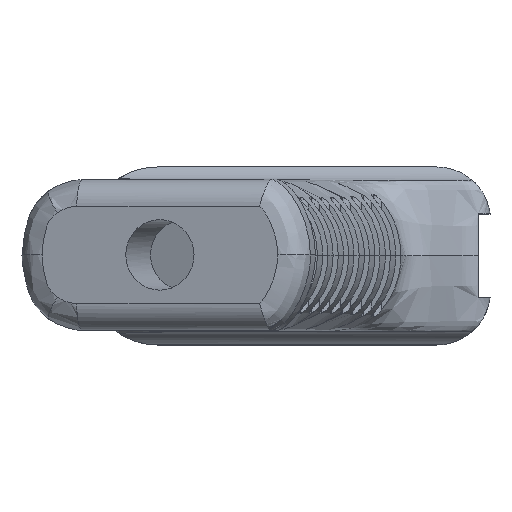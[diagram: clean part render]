
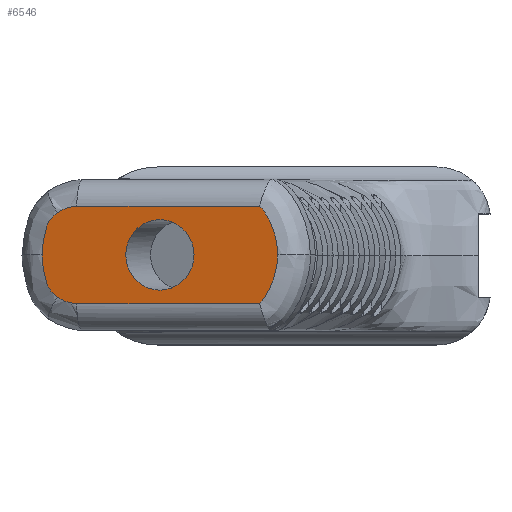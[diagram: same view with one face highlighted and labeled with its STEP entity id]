
A CAD part, top view. The second image highlights one B-rep face of the part: STEP entity #6546.
In plain terms, the highlighted planar face has unit normal (-0.249, 0, 0.969).
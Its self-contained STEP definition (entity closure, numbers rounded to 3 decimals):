
#104=B_SPLINE_CURVE_WITH_KNOTS('',3,(#9156,#9157,#9158,#9159,#9160,#9161,
#9162,#9163,#9164,#9165,#9166,#9167,#9168,#9169,#9170,#9171,#9172,#9173,
#9174,#9175,#9176,#9177,#9178),.UNSPECIFIED.,.F.,.F.,(4,1,1,1,1,1,2,1,1,
1,1,1,2,1,2,1,1,4),(0.,0.054,0.161,
0.214,0.268,0.321,0.375,
0.444,0.513,0.582,0.651,
0.685,0.72,0.745,0.761,
0.775,0.788,0.793),.UNSPECIFIED.);
#105=B_SPLINE_CURVE_WITH_KNOTS('',3,(#9180,#9181,#9182,#9183,#9184,#9185,
#9186,#9187,#9188,#9189,#9190,#9191,#9192,#9193,#9194),.UNSPECIFIED.,.F.,
 .F.,(4,1,1,1,1,1,1,1,2,1,1,4),(0.035,0.044,0.066,
0.08,0.108,0.223,0.338,
0.395,0.453,0.578,0.703,
0.828),.UNSPECIFIED.);
#106=B_SPLINE_CURVE_WITH_KNOTS('',3,(#9198,#9199,#9200,#9201,#9202,#9203),
 .UNSPECIFIED.,.F.,.F.,(4,2,4),(-0.321,-0.296,-0.005),
 .UNSPECIFIED.);
#107=B_SPLINE_CURVE_WITH_KNOTS('',3,(#9205,#9206,#9207,#9208,#9209,#9210,
#9211,#9212),.UNSPECIFIED.,.F.,.F.,(4,1,2,1,4),(0.,0.25,0.438,
0.549,0.696),.UNSPECIFIED.);
#108=B_SPLINE_CURVE_WITH_KNOTS('',3,(#9214,#9215,#9216,#9217,#9218,#9219,
#9220),.UNSPECIFIED.,.F.,.F.,(4,1,2,4),(0.,0.148,0.26,
0.698),.UNSPECIFIED.);
#109=B_SPLINE_CURVE_WITH_KNOTS('',3,(#9221,#9222,#9223,#9224,#9225,#9226),
 .UNSPECIFIED.,.F.,.F.,(4,2,4),(-0.316,-0.025,
0.),.UNSPECIFIED.);
#658=FACE_BOUND('',#1186,.T.);
#667=CIRCLE('',#6907,5.25);
#814=FACE_OUTER_BOUND('',#1185,.T.);
#1185=EDGE_LOOP('',(#4716,#4717,#4718,#4719,#4720,#4721,#4722,#4723));
#1186=EDGE_LOOP('',(#4724));
#1679=LINE('',#9154,#2199);
#1680=LINE('',#9196,#2200);
#2199=VECTOR('',#7694,10.);
#2200=VECTOR('',#7695,10.);
#2630=VERTEX_POINT('',#8848);
#2690=VERTEX_POINT('',#9152);
#2691=VERTEX_POINT('',#9153);
#2692=VERTEX_POINT('',#9155);
#2693=VERTEX_POINT('',#9179);
#2694=VERTEX_POINT('',#9195);
#2695=VERTEX_POINT('',#9197);
#2696=VERTEX_POINT('',#9204);
#2697=VERTEX_POINT('',#9213);
#3358=EDGE_CURVE('',#2630,#2630,#667,.T.);
#3448=EDGE_CURVE('',#2690,#2691,#1679,.T.);
#3449=EDGE_CURVE('',#2692,#2690,#104,.T.);
#3450=EDGE_CURVE('',#2693,#2692,#105,.T.);
#3451=EDGE_CURVE('',#2694,#2693,#1680,.T.);
#3452=EDGE_CURVE('',#2695,#2694,#106,.T.);
#3453=EDGE_CURVE('',#2696,#2695,#107,.T.);
#3454=EDGE_CURVE('',#2697,#2696,#108,.T.);
#3455=EDGE_CURVE('',#2691,#2697,#109,.T.);
#4716=ORIENTED_EDGE('',*,*,#3448,.F.);
#4717=ORIENTED_EDGE('',*,*,#3449,.F.);
#4718=ORIENTED_EDGE('',*,*,#3450,.F.);
#4719=ORIENTED_EDGE('',*,*,#3451,.F.);
#4720=ORIENTED_EDGE('',*,*,#3452,.F.);
#4721=ORIENTED_EDGE('',*,*,#3453,.F.);
#4722=ORIENTED_EDGE('',*,*,#3454,.F.);
#4723=ORIENTED_EDGE('',*,*,#3455,.F.);
#4724=ORIENTED_EDGE('',*,*,#3358,.T.);
#6342=PLANE('',#6974);
#6546=ADVANCED_FACE('',(#814,#658),#6342,.F.);
#6907=AXIS2_PLACEMENT_3D('',#8849,#7508,#7509);
#6974=AXIS2_PLACEMENT_3D('',#9151,#7692,#7693);
#7508=DIRECTION('center_axis',(0.249,0.,-0.969));
#7509=DIRECTION('ref_axis',(0.,-1.,0.));
#7692=DIRECTION('center_axis',(0.249,0.,-0.969));
#7693=DIRECTION('ref_axis',(0.969,0.,0.249));
#7694=DIRECTION('',(-0.969,0.,-0.249));
#7695=DIRECTION('',(0.969,0.,0.249));
#8848=CARTESIAN_POINT('',(-49.151,-78.684,-18.57));
#8849=CARTESIAN_POINT('Origin',(-49.151,-83.934,-18.57));
#9151=CARTESIAN_POINT('Origin',(-81.64,-72.686,-26.907));
#9152=CARTESIAN_POINT('',(-34.333,-91.182,-14.767));
#9153=CARTESIAN_POINT('',(-61.522,-91.18,-21.745));
#9154=CARTESIAN_POINT('',(-52.784,-91.182,-19.502));
#9155=CARTESIAN_POINT('',(-31.61,-83.935,-14.069));
#9156=CARTESIAN_POINT('Ctrl Pts',(-31.61,-83.935,-14.069));
#9157=CARTESIAN_POINT('Ctrl Pts',(-31.61,-84.112,-14.069));
#9158=CARTESIAN_POINT('Ctrl Pts',(-31.625,-84.648,-14.072));
#9159=CARTESIAN_POINT('Ctrl Pts',(-31.699,-85.362,-14.091));
#9160=CARTESIAN_POINT('Ctrl Pts',(-31.825,-86.069,-14.124));
#9161=CARTESIAN_POINT('Ctrl Pts',(-31.945,-86.593,-14.154));
#9162=CARTESIAN_POINT('Ctrl Pts',(-32.089,-87.109,-14.192));
#9163=CARTESIAN_POINT('Ctrl Pts',(-32.201,-87.447,-14.22));
#9164=CARTESIAN_POINT('Ctrl Pts',(-32.34,-87.83,-14.256));
#9165=CARTESIAN_POINT('Ctrl Pts',(-32.504,-88.26,-14.298));
#9166=CARTESIAN_POINT('Ctrl Pts',(-32.777,-88.892,-14.368));
#9167=CARTESIAN_POINT('Ctrl Pts',(-33.083,-89.509,-14.447));
#9168=CARTESIAN_POINT('Ctrl Pts',(-33.368,-90.002,-14.52));
#9169=CARTESIAN_POINT('Ctrl Pts',(-33.623,-90.384,-14.585));
#9170=CARTESIAN_POINT('Ctrl Pts',(-33.761,-90.569,-14.62));
#9171=CARTESIAN_POINT('Ctrl Pts',(-33.884,-90.723,-14.652));
#9172=CARTESIAN_POINT('Ctrl Pts',(-33.972,-90.828,-14.675));
#9173=CARTESIAN_POINT('Ctrl Pts',(-34.065,-90.929,-14.699));
#9174=CARTESIAN_POINT('Ctrl Pts',(-34.133,-90.999,-14.716));
#9175=CARTESIAN_POINT('Ctrl Pts',(-34.195,-91.061,-14.732));
#9176=CARTESIAN_POINT('Ctrl Pts',(-34.273,-91.131,-14.752));
#9177=CARTESIAN_POINT('Ctrl Pts',(-34.319,-91.17,-14.764));
#9178=CARTESIAN_POINT('Ctrl Pts',(-34.333,-91.182,-14.767));
#9179=CARTESIAN_POINT('',(-34.333,-76.686,-14.767));
#9180=CARTESIAN_POINT('Ctrl Pts',(-34.333,-76.686,-14.767));
#9181=CARTESIAN_POINT('Ctrl Pts',(-34.308,-76.706,-14.761));
#9182=CARTESIAN_POINT('Ctrl Pts',(-34.229,-76.775,-14.741));
#9183=CARTESIAN_POINT('Ctrl Pts',(-34.121,-76.879,-14.713));
#9184=CARTESIAN_POINT('Ctrl Pts',(-33.977,-77.033,-14.676));
#9185=CARTESIAN_POINT('Ctrl Pts',(-33.646,-77.428,-14.591));
#9186=CARTESIAN_POINT('Ctrl Pts',(-33.185,-78.145,-14.473));
#9187=CARTESIAN_POINT('Ctrl Pts',(-32.759,-79.006,-14.363));
#9188=CARTESIAN_POINT('Ctrl Pts',(-32.462,-79.717,-14.287));
#9189=CARTESIAN_POINT('Ctrl Pts',(-32.326,-80.074,-14.252));
#9190=CARTESIAN_POINT('Ctrl Pts',(-32.121,-80.645,-14.2));
#9191=CARTESIAN_POINT('Ctrl Pts',(-31.883,-81.447,-14.139));
#9192=CARTESIAN_POINT('Ctrl Pts',(-31.662,-82.68,-14.082));
#9193=CARTESIAN_POINT('Ctrl Pts',(-31.61,-83.517,-14.069));
#9194=CARTESIAN_POINT('Ctrl Pts',(-31.61,-83.935,-14.069));
#9195=CARTESIAN_POINT('',(-61.522,-76.686,-21.745));
#9196=CARTESIAN_POINT('',(-52.784,-76.686,-19.502));
#9197=CARTESIAN_POINT('',(-64.4,-77.649,-22.483));
#9198=CARTESIAN_POINT('Ctrl Pts',(-64.4,-77.649,-22.483));
#9199=CARTESIAN_POINT('Ctrl Pts',(-64.332,-77.602,-22.466));
#9200=CARTESIAN_POINT('Ctrl Pts',(-64.264,-77.557,-22.448));
#9201=CARTESIAN_POINT('Ctrl Pts',(-63.391,-77.01,-22.224));
#9202=CARTESIAN_POINT('Ctrl Pts',(-62.461,-76.72,-21.986));
#9203=CARTESIAN_POINT('Ctrl Pts',(-61.522,-76.689,-21.745));
#9204=CARTESIAN_POINT('',(-66.692,-83.934,-23.071));
#9205=CARTESIAN_POINT('Ctrl Pts',(-66.692,-83.934,-23.071));
#9206=CARTESIAN_POINT('Ctrl Pts',(-66.692,-83.101,-23.071));
#9207=CARTESIAN_POINT('Ctrl Pts',(-66.542,-81.632,-23.033));
#9208=CARTESIAN_POINT('Ctrl Pts',(-66.167,-80.221,-22.937));
#9209=CARTESIAN_POINT('Ctrl Pts',(-65.858,-79.27,-22.857));
#9210=CARTESIAN_POINT('Ctrl Pts',(-65.438,-78.517,-22.749));
#9211=CARTESIAN_POINT('Ctrl Pts',(-64.796,-77.925,-22.585));
#9212=CARTESIAN_POINT('Ctrl Pts',(-64.4,-77.649,-22.483));
#9213=CARTESIAN_POINT('',(-64.4,-90.218,-22.483));
#9214=CARTESIAN_POINT('Ctrl Pts',(-64.4,-90.218,-22.483));
#9215=CARTESIAN_POINT('Ctrl Pts',(-64.797,-89.942,-22.585));
#9216=CARTESIAN_POINT('Ctrl Pts',(-65.433,-89.357,-22.748));
#9217=CARTESIAN_POINT('Ctrl Pts',(-65.858,-88.597,-22.857));
#9218=CARTESIAN_POINT('Ctrl Pts',(-66.423,-86.86,-23.002));
#9219=CARTESIAN_POINT('Ctrl Pts',(-66.692,-85.395,-23.071));
#9220=CARTESIAN_POINT('Ctrl Pts',(-66.692,-83.934,-23.071));
#9221=CARTESIAN_POINT('Ctrl Pts',(-61.522,-91.179,-21.745));
#9222=CARTESIAN_POINT('Ctrl Pts',(-62.461,-91.148,-21.986));
#9223=CARTESIAN_POINT('Ctrl Pts',(-63.391,-90.858,-22.224));
#9224=CARTESIAN_POINT('Ctrl Pts',(-64.264,-90.311,-22.448));
#9225=CARTESIAN_POINT('Ctrl Pts',(-64.332,-90.265,-22.466));
#9226=CARTESIAN_POINT('Ctrl Pts',(-64.4,-90.218,-22.483));
